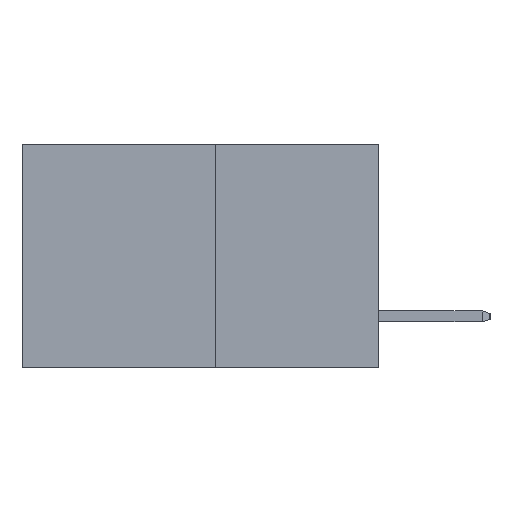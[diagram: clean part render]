
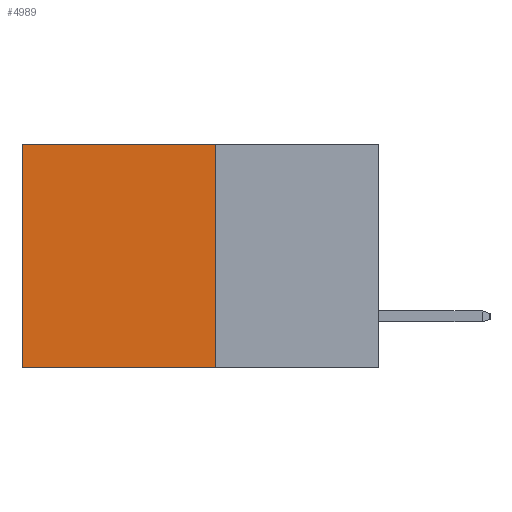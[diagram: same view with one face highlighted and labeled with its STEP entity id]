
A CAD part, left-side view. The second image highlights one B-rep face of the part: STEP entity #4989.
In plain terms, the highlighted planar face has unit normal (-1, 0, 0).
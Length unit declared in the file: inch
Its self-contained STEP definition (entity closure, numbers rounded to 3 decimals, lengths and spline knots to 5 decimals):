
#207 = LINE ( 'NONE', #8849, #5889 ) ;
#427 = CARTESIAN_POINT ( 'NONE',  ( 0.277, 0.27, -0.37 ) ) ;
#852 = PLANE ( 'NONE',  #3199 ) ;
#1068 = CARTESIAN_POINT ( 'NONE',  ( 0.277, 0.27, -0.37 ) ) ;
#1474 = VERTEX_POINT ( 'NONE', #427 ) ;
#1737 = ORIENTED_EDGE ( 'NONE', *, *, #7102, .T. ) ;
#1743 = DIRECTION ( 'NONE',  ( 0., 1., 0. ) ) ;
#1776 = CARTESIAN_POINT ( 'NONE',  ( 0.277, 0.27, -0.37 ) ) ;
#2024 = VECTOR ( 'NONE', #1743, 39.37008 ) ;
#2261 = LINE ( 'NONE', #1776, #2024 ) ;
#2291 = LINE ( 'NONE', #5431, #7408 ) ;
#2318 = ORIENTED_EDGE ( 'NONE', *, *, #8373, .F. ) ;
#2417 = ORIENTED_EDGE ( 'NONE', *, *, #3869, .T. ) ;
#3067 = VECTOR ( 'NONE', #6457, 39.37008 ) ;
#3199 = AXIS2_PLACEMENT_3D ( 'NONE', #3206, #5484, #5971 ) ;
#3206 = CARTESIAN_POINT ( 'NONE',  ( 0.277, 0.27, -0.37 ) ) ;
#3869 = EDGE_CURVE ( 'NONE', #5215, #5522, #207, .T. ) ;
#4376 = CARTESIAN_POINT ( 'NONE',  ( 0.277, 0.59, 0. ) ) ;
#4989 = ADVANCED_FACE ( 'NONE', ( #5218 ), #852, .F. ) ;
#4990 = EDGE_LOOP ( 'NONE', ( #2417, #7339, #2318, #1737 ) ) ;
#5031 = CARTESIAN_POINT ( 'NONE',  ( 0.277, 0.27, 0. ) ) ;
#5215 = VERTEX_POINT ( 'NONE', #4376 ) ;
#5218 = FACE_OUTER_BOUND ( 'NONE', #4990, .T. ) ;
#5354 = DIRECTION ( 'NONE',  ( 0., 1., 0. ) ) ;
#5431 = CARTESIAN_POINT ( 'NONE',  ( 0.277, 0.27, 0. ) ) ;
#5464 = CARTESIAN_POINT ( 'NONE',  ( 0.277, 0.59, -0.37 ) ) ;
#5484 = DIRECTION ( 'NONE',  ( 1., 0., 0. ) ) ;
#5522 = VERTEX_POINT ( 'NONE', #5464 ) ;
#5889 = VECTOR ( 'NONE', #8022, 39.37008 ) ;
#5971 = DIRECTION ( 'NONE',  ( 0., 0., -1. ) ) ;
#6457 = DIRECTION ( 'NONE',  ( 0., 0., -1. ) ) ;
#6738 = VERTEX_POINT ( 'NONE', #5031 ) ;
#6935 = LINE ( 'NONE', #1068, #3067 ) ;
#7102 = EDGE_CURVE ( 'NONE', #6738, #5215, #2291, .T. ) ;
#7339 = ORIENTED_EDGE ( 'NONE', *, *, #8273, .F. ) ;
#7408 = VECTOR ( 'NONE', #5354, 39.37008 ) ;
#8022 = DIRECTION ( 'NONE',  ( 0., 0., -1. ) ) ;
#8273 = EDGE_CURVE ( 'NONE', #1474, #5522, #2261, .T. ) ;
#8373 = EDGE_CURVE ( 'NONE', #6738, #1474, #6935, .T. ) ;
#8849 = CARTESIAN_POINT ( 'NONE',  ( 0.277, 0.59, -0.37 ) ) ;
